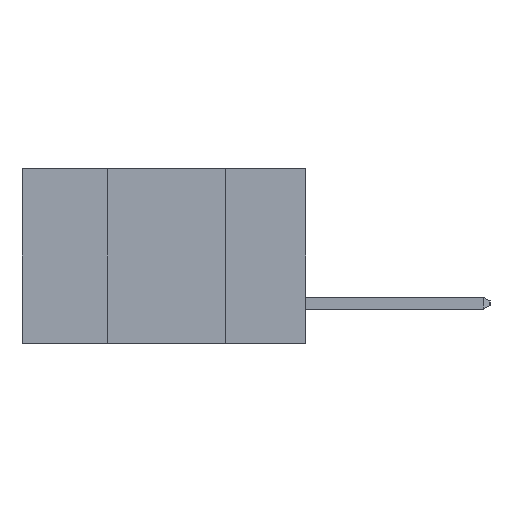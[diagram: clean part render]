
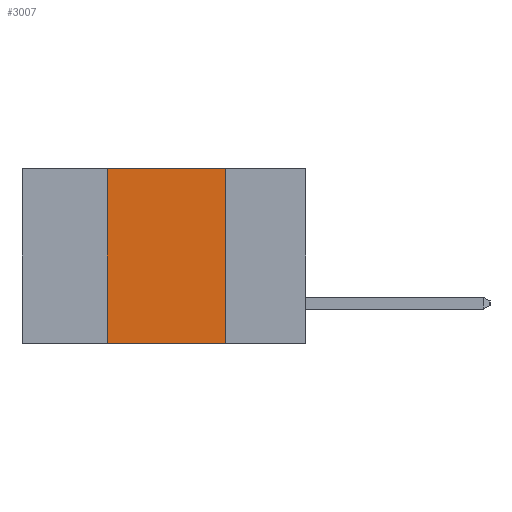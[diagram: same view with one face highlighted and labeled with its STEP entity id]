
A CAD part, left-side view. The second image highlights one B-rep face of the part: STEP entity #3007.
In plain terms, the highlighted planar face has unit normal (-1, 0, 0).
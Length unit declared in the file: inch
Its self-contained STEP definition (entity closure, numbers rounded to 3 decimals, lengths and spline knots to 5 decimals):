
#45 = CARTESIAN_POINT ( 'NONE',  ( 0., 0.6, 0. ) ) ;
#58 = DIRECTION ( 'NONE',  ( 0., -1., 0. ) ) ;
#211 = PLANE ( 'NONE',  #1933 ) ;
#676 = FACE_OUTER_BOUND ( 'NONE', #9285, .T. ) ;
#1008 = EDGE_CURVE ( 'NONE', #5618, #1778, #7094, .T. ) ;
#1368 = DIRECTION ( 'NONE',  ( 0., 0., -1. ) ) ;
#1443 = DIRECTION ( 'NONE',  ( 0., 0., 1. ) ) ;
#1517 = CARTESIAN_POINT ( 'NONE',  ( 0., 0.42, -0.37 ) ) ;
#1628 = EDGE_CURVE ( 'NONE', #5618, #6239, #12049, .T. ) ;
#1778 = VERTEX_POINT ( 'NONE', #9885 ) ;
#1933 = AXIS2_PLACEMENT_3D ( 'NONE', #10780, #10925, #10934 ) ;
#2518 = CARTESIAN_POINT ( 'NONE',  ( 0., 0.42, -0.37 ) ) ;
#2546 = EDGE_CURVE ( 'NONE', #3580, #1778, #3330, .T. ) ;
#2560 = VECTOR ( 'NONE', #1443, 39.37008 ) ;
#3007 = ADVANCED_FACE ( 'NONE', ( #676 ), #211, .F. ) ;
#3032 = VECTOR ( 'NONE', #1368, 39.37008 ) ;
#3330 = LINE ( 'NONE', #12030, #3032 ) ;
#3580 = VERTEX_POINT ( 'NONE', #8557 ) ;
#3667 = ORIENTED_EDGE ( 'NONE', *, *, #1008, .T. ) ;
#4411 = VECTOR ( 'NONE', #9666, 39.37008 ) ;
#4506 = EDGE_CURVE ( 'NONE', #6239, #3580, #10536, .T. ) ;
#5267 = ORIENTED_EDGE ( 'NONE', *, *, #2546, .F. ) ;
#5525 = ORIENTED_EDGE ( 'NONE', *, *, #1628, .F. ) ;
#5618 = VERTEX_POINT ( 'NONE', #2518 ) ;
#5637 = VECTOR ( 'NONE', #58, 39.37008 ) ;
#6239 = VERTEX_POINT ( 'NONE', #9912 ) ;
#7094 = LINE ( 'NONE', #9140, #4411 ) ;
#8083 = ORIENTED_EDGE ( 'NONE', *, *, #4506, .F. ) ;
#8557 = CARTESIAN_POINT ( 'NONE',  ( 0., 0.17, 0. ) ) ;
#9140 = CARTESIAN_POINT ( 'NONE',  ( 0., 0.6, -0.37 ) ) ;
#9285 = EDGE_LOOP ( 'NONE', ( #5267, #8083, #5525, #3667 ) ) ;
#9666 = DIRECTION ( 'NONE',  ( 0., -1., 0. ) ) ;
#9885 = CARTESIAN_POINT ( 'NONE',  ( 0., 0.17, -0.37 ) ) ;
#9912 = CARTESIAN_POINT ( 'NONE',  ( 0., 0.42, 0. ) ) ;
#10536 = LINE ( 'NONE', #45, #5637 ) ;
#10780 = CARTESIAN_POINT ( 'NONE',  ( 0., 0.6, 0. ) ) ;
#10925 = DIRECTION ( 'NONE',  ( 1., 0., 0. ) ) ;
#10934 = DIRECTION ( 'NONE',  ( 0., 0., -1. ) ) ;
#12030 = CARTESIAN_POINT ( 'NONE',  ( 0., 0.17, -0.37 ) ) ;
#12049 = LINE ( 'NONE', #1517, #2560 ) ;
